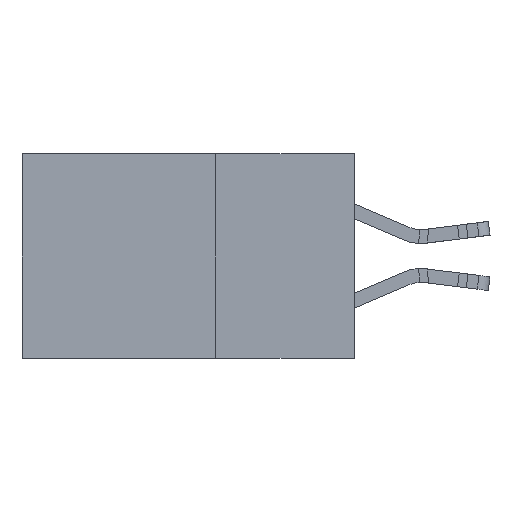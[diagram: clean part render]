
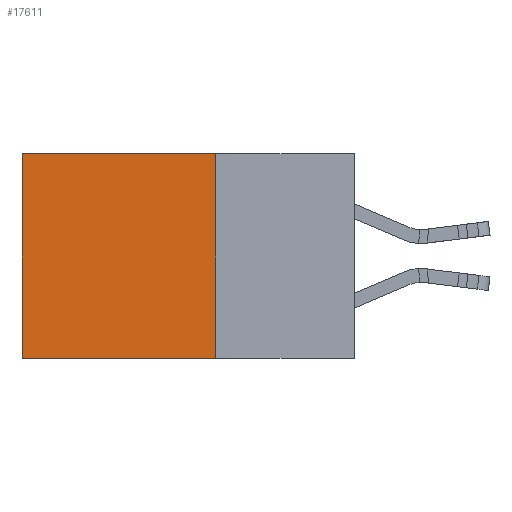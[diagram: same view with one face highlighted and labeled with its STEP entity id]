
A CAD part, left-side view. The second image highlights one B-rep face of the part: STEP entity #17611.
In plain terms, the highlighted planar face has unit normal (-1, 0, 0).
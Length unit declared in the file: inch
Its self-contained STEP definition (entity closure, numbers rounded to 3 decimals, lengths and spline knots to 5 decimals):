
#73 = VERTEX_POINT ( 'NONE', #21429 ) ;
#1266 = LINE ( 'NONE', #7373, #13108 ) ;
#1700 = CARTESIAN_POINT ( 'NONE',  ( 0.2615, 0.25, -0.37 ) ) ;
#1932 = LINE ( 'NONE', #24340, #25180 ) ;
#3460 = ORIENTED_EDGE ( 'NONE', *, *, #25212, .F. ) ;
#3744 = DIRECTION ( 'NONE',  ( 0., 0., -1. ) ) ;
#4141 = DIRECTION ( 'NONE',  ( 1., 0., 0. ) ) ;
#6987 = CARTESIAN_POINT ( 'NONE',  ( 0.2615, 0.6, -0.37 ) ) ;
#7373 = CARTESIAN_POINT ( 'NONE',  ( 0.2615, 0.25, -0.37 ) ) ;
#7409 = EDGE_CURVE ( 'NONE', #15846, #9861, #7812, .T. ) ;
#7812 = LINE ( 'NONE', #24633, #16172 ) ;
#7866 = CARTESIAN_POINT ( 'NONE',  ( 0.2615, 0.25, 0. ) ) ;
#8062 = VECTOR ( 'NONE', #17528, 39.37008 ) ;
#8968 = AXIS2_PLACEMENT_3D ( 'NONE', #11853, #4141, #3744 ) ;
#9861 = VERTEX_POINT ( 'NONE', #6987 ) ;
#9913 = ORIENTED_EDGE ( 'NONE', *, *, #17227, .T. ) ;
#11669 = LINE ( 'NONE', #1700, #8062 ) ;
#11853 = CARTESIAN_POINT ( 'NONE',  ( 0.2615, 0.25, -0.37 ) ) ;
#13108 = VECTOR ( 'NONE', #15479, 39.37008 ) ;
#15479 = DIRECTION ( 'NONE',  ( 0., 0., -1. ) ) ;
#15846 = VERTEX_POINT ( 'NONE', #18906 ) ;
#15969 = FACE_OUTER_BOUND ( 'NONE', #21518, .T. ) ;
#16037 = EDGE_CURVE ( 'NONE', #73, #9861, #11669, .T. ) ;
#16172 = VECTOR ( 'NONE', #26274, 39.37008 ) ;
#16729 = VERTEX_POINT ( 'NONE', #7866 ) ;
#17227 = EDGE_CURVE ( 'NONE', #16729, #15846, #1932, .T. ) ;
#17528 = DIRECTION ( 'NONE',  ( 0., 1., 0. ) ) ;
#17611 = ADVANCED_FACE ( 'NONE', ( #15969 ), #26323, .F. ) ;
#18296 = DIRECTION ( 'NONE',  ( 0., 1., 0. ) ) ;
#18906 = CARTESIAN_POINT ( 'NONE',  ( 0.2615, 0.6, 0. ) ) ;
#19380 = ORIENTED_EDGE ( 'NONE', *, *, #16037, .F. ) ;
#20891 = ORIENTED_EDGE ( 'NONE', *, *, #7409, .T. ) ;
#21429 = CARTESIAN_POINT ( 'NONE',  ( 0.2615, 0.25, -0.37 ) ) ;
#21518 = EDGE_LOOP ( 'NONE', ( #20891, #19380, #3460, #9913 ) ) ;
#24340 = CARTESIAN_POINT ( 'NONE',  ( 0.2615, 0.25, 0. ) ) ;
#24633 = CARTESIAN_POINT ( 'NONE',  ( 0.2615, 0.6, -0.37 ) ) ;
#25180 = VECTOR ( 'NONE', #18296, 39.37008 ) ;
#25212 = EDGE_CURVE ( 'NONE', #16729, #73, #1266, .T. ) ;
#26274 = DIRECTION ( 'NONE',  ( 0., 0., -1. ) ) ;
#26323 = PLANE ( 'NONE',  #8968 ) ;
